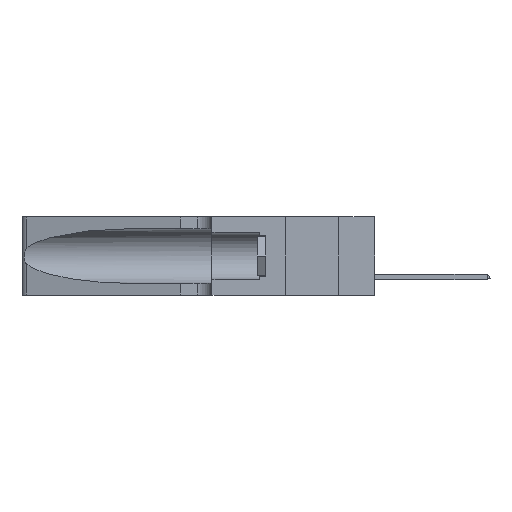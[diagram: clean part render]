
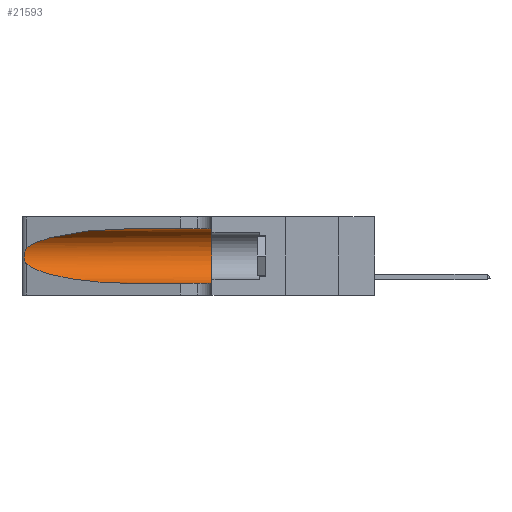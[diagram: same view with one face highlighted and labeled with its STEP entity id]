
A CAD part, left-side view. The second image highlights one B-rep face of the part: STEP entity #21593.
In plain terms, the highlighted cylindrical face has radius 3.308 mm (diameter 6.617 mm), a partial arc.
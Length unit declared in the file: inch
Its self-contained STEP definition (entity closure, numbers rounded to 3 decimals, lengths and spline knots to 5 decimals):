
#195 = CIRCLE ( 'NONE', #25286, 0.13025 ) ;
#1002 = CARTESIAN_POINT ( 'NONE',  ( 0.25487, 1.22718, 0.22369 ) ) ;
#1104 = CARTESIAN_POINT ( 'NONE',  ( 0.25555, 1.22994, 0.2215 ) ) ;
#1351 = CARTESIAN_POINT ( 'NONE',  ( 0.1305, 0.72297, 0.31525 ) ) ;
#1512 = DIRECTION ( 'NONE',  ( 0., -1., 0. ) ) ;
#1692 = VERTEX_POINT ( 'NONE', #18161 ) ;
#2673 = ORIENTED_EDGE ( 'NONE', *, *, #16457, .T. ) ;
#4961 = VERTEX_POINT ( 'NONE', #6443 ) ;
#5287 = VERTEX_POINT ( 'NONE', #6758 ) ;
#5730 = CARTESIAN_POINT ( 'NONE',  ( 0.2373, 1.15595, 0.08982 ) ) ;
#6107 = CARTESIAN_POINT ( 'NONE',  ( 0.18966, 0.96281, 0.05475 ) ) ;
#6443 = CARTESIAN_POINT ( 'NONE',  ( 0.25487, 1.22718, 0.22369 ) ) ;
#6530 = CARTESIAN_POINT ( 'NONE',  ( 0.25487, 1.22718, 0.14631 ) ) ;
#6556 = ORIENTED_EDGE ( 'NONE', *, *, #13511, .T. ) ;
#6758 = CARTESIAN_POINT ( 'NONE',  ( 0.1305, 0.35, 0.05475 ) ) ;
#7140 = CARTESIAN_POINT ( 'NONE',  ( 0.1305, 0.72297, 0.05475 ) ) ;
#7689 = FACE_OUTER_BOUND ( 'NONE', #26531, .T. ) ;
#7969 = DIRECTION ( 'NONE',  ( 0., -1., 0. ) ) ;
#8332 = DIRECTION ( 'NONE',  ( 0., 0., -1. ) ) ;
#8465 = EDGE_CURVE ( 'NONE', #1692, #4961, #20361, .T. ) ;
#8639 = EDGE_CURVE ( 'NONE', #27257, #5287, #195, .T. ) ;
#8849 = EDGE_CURVE ( 'NONE', #1692, #27257, #19054, .T. ) ;
#9712 = EDGE_CURVE ( 'NONE', #12670, #5287, #22074, .T. ) ;
#9952 = ORIENTED_EDGE ( 'NONE', *, *, #8849, .F. ) ;
#9971 = CARTESIAN_POINT ( 'NONE',  ( 0.25639, 1.23184, 0.21858 ) ) ;
#10027 = CARTESIAN_POINT ( 'NONE',  ( 0.2373, 1.15595, 0.28018 ) ) ;
#10172 = CARTESIAN_POINT ( 'NONE',  ( 0.25787, 1.23484, 0.2124 ) ) ;
#10727 = CARTESIAN_POINT ( 'NONE',  ( 0.25854, 1.2359, 0.20912 ) ) ;
#11058 = CARTESIAN_POINT ( 'NONE',  ( 0.1305, 0.35, 0.185 ) ) ;
#11813 = CARTESIAN_POINT ( 'NONE',  ( 0.25487, 1.22718, 0.14631 ) ) ;
#12431 = CARTESIAN_POINT ( 'NONE',  ( 0.1305, 1.61858, 0.31525 ) ) ;
#12670 = VERTEX_POINT ( 'NONE', #7140 ) ;
#12845 = DIRECTION ( 'NONE',  ( 0., -1., 0. ) ) ;
#12992 = DIRECTION ( 'NONE',  ( 0., 0., 1. ) ) ;
#13213 = VECTOR ( 'NONE', #1512, 39.37008 ) ;
#13283 = DIRECTION ( 'NONE',  ( 0., 1., 0. ) ) ;
#13511 = EDGE_CURVE ( 'NONE', #4961, #23655, #24242, .T. ) ;
#14118 = CARTESIAN_POINT ( 'NONE',  ( 0.1305, 1.61858, 0.05475 ) ) ;
#14829 = CARTESIAN_POINT ( 'NONE',  ( 0.1305, 0.72297, 0.05475 ) ) ;
#15620 = ORIENTED_EDGE ( 'NONE', *, *, #9712, .T. ) ;
#15731 = CARTESIAN_POINT ( 'NONE',  ( 0.26017, 1.23833, 0.17102 ) ) ;
#16457 = EDGE_CURVE ( 'NONE', #23655, #12670, #18254, .T. ) ;
#17007 = ORIENTED_EDGE ( 'NONE', *, *, #8639, .F. ) ;
#17579 = CARTESIAN_POINT ( 'NONE',  ( 0.25639, 1.23186, 0.15144 ) ) ;
#17689 = CARTESIAN_POINT ( 'NONE',  ( 0.1305, 0.35, 0.31525 ) ) ;
#18161 = CARTESIAN_POINT ( 'NONE',  ( 0.1305, 0.72297, 0.31525 ) ) ;
#18254 =( BOUNDED_CURVE ( )  B_SPLINE_CURVE ( 3, ( #19226, #5730, #6107, #14829 ),
 .UNSPECIFIED., .F., .F. ) 
 B_SPLINE_CURVE_WITH_KNOTS ( ( 4, 4 ),
 ( 3.44316, 4.71239 ),
 .UNSPECIFIED. ) 
 CURVE ( )  GEOMETRIC_REPRESENTATION_ITEM ( )  RATIONAL_B_SPLINE_CURVE ( ( 1., 0.87, 0.87, 1. ) ) 
 REPRESENTATION_ITEM ( '' )  );
#19054 = LINE ( 'NONE', #12431, #13213 ) ;
#19226 = CARTESIAN_POINT ( 'NONE',  ( 0.25487, 1.22718, 0.14631 ) ) ;
#19360 = CARTESIAN_POINT ( 'NONE',  ( 0.18966, 0.96281, 0.31525 ) ) ;
#19390 = CARTESIAN_POINT ( 'NONE',  ( 0.26075, 1.23896, 0.19203 ) ) ;
#19570 = CARTESIAN_POINT ( 'NONE',  ( 0.26018, 1.23835, 0.19895 ) ) ;
#19962 = CARTESIAN_POINT ( 'NONE',  ( 0.25555, 1.22993, 0.14849 ) ) ;
#19990 = VECTOR ( 'NONE', #7969, 39.37008 ) ;
#20361 =( BOUNDED_CURVE ( )  B_SPLINE_CURVE ( 3, ( #1351, #19360, #10027, #25382 ),
 .UNSPECIFIED., .F., .F. ) 
 B_SPLINE_CURVE_WITH_KNOTS ( ( 4, 4 ),
 ( 1.5708, 2.84003 ),
 .UNSPECIFIED. ) 
 CURVE ( )  GEOMETRIC_REPRESENTATION_ITEM ( )  RATIONAL_B_SPLINE_CURVE ( ( 1., 0.87, 0.87, 1. ) ) 
 REPRESENTATION_ITEM ( '' )  );
#21593 = ADVANCED_FACE ( 'NONE', ( #7689 ), #27581, .F. ) ;
#22074 = LINE ( 'NONE', #14118, #19990 ) ;
#22230 = AXIS2_PLACEMENT_3D ( 'NONE', #27606, #12845, #8332 ) ;
#23655 = VERTEX_POINT ( 'NONE', #6530 ) ;
#23961 = ORIENTED_EDGE ( 'NONE', *, *, #8465, .T. ) ;
#24242 = B_SPLINE_CURVE_WITH_KNOTS ( 'NONE', 3,
 ( #1002, #1104, #9971, #10172, #10727, #19570, #19390, #25784, #15731, #26643, #26371, #17579, #19962, #11813 ),
 .UNSPECIFIED., .F., .F.,
 ( 4, 2, 2, 2, 2, 2, 4 ),
 ( 0., 0.00027, 0.00053, 0.00107, 0.0016, 0.00187, 0.00214 ),
 .UNSPECIFIED. ) ;
#25286 = AXIS2_PLACEMENT_3D ( 'NONE', #11058, #13283, #12992 ) ;
#25382 = CARTESIAN_POINT ( 'NONE',  ( 0.25487, 1.22718, 0.22369 ) ) ;
#25784 = CARTESIAN_POINT ( 'NONE',  ( 0.26075, 1.23896, 0.178 ) ) ;
#26371 = CARTESIAN_POINT ( 'NONE',  ( 0.25789, 1.23486, 0.15765 ) ) ;
#26531 = EDGE_LOOP ( 'NONE', ( #23961, #6556, #2673, #15620, #17007, #9952 ) ) ;
#26643 = CARTESIAN_POINT ( 'NONE',  ( 0.25856, 1.23593, 0.16098 ) ) ;
#27257 = VERTEX_POINT ( 'NONE', #17689 ) ;
#27581 = CYLINDRICAL_SURFACE ( 'NONE', #22230, 0.13025 ) ;
#27606 = CARTESIAN_POINT ( 'NONE',  ( 0.1305, 1.61858, 0.185 ) ) ;
